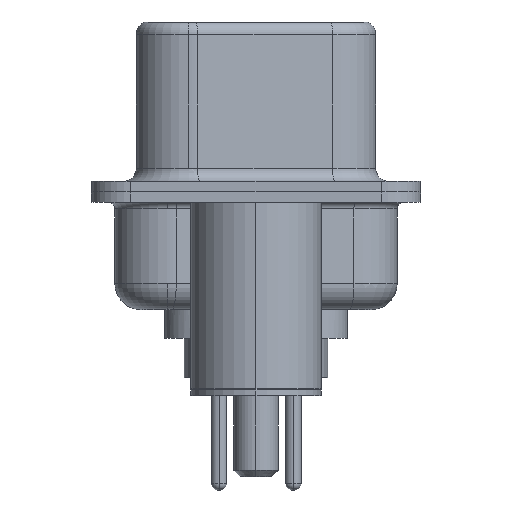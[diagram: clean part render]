
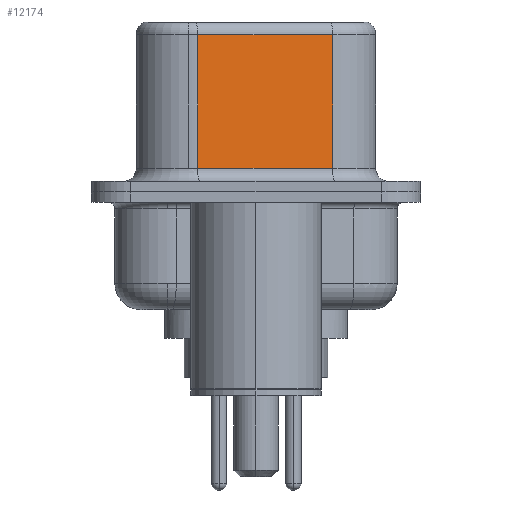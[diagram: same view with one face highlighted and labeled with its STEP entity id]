
A CAD part, left-side view. The second image highlights one B-rep face of the part: STEP entity #12174.
In plain terms, the highlighted planar face has unit normal (-0.985, -0.174, 0).
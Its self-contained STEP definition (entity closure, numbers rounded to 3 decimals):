
#230 = DIRECTION ( 'NONE',  ( 0.174, -0.985, 0. ) ) ;
#518 = CARTESIAN_POINT ( 'NONE',  ( 3.655, 2.233, 0.9 ) ) ;
#593 = VERTEX_POINT ( 'NONE', #15364 ) ;
#1044 = CARTESIAN_POINT ( 'NONE',  ( 4.565, -2.927, 6.02 ) ) ;
#1644 = CARTESIAN_POINT ( 'NONE',  ( 4.565, -2.927, 6.02 ) ) ;
#1929 = CARTESIAN_POINT ( 'NONE',  ( 3.655, 2.233, 6.02 ) ) ;
#2611 = ORIENTED_EDGE ( 'NONE', *, *, #14477, .T. ) ;
#2625 = CARTESIAN_POINT ( 'NONE',  ( 4.565, -2.927, 6.52 ) ) ;
#2682 = EDGE_CURVE ( 'NONE', #6691, #593, #7657, .T. ) ;
#3186 = ORIENTED_EDGE ( 'NONE', *, *, #2682, .F. ) ;
#3471 = AXIS2_PLACEMENT_3D ( 'NONE', #12317, #14825, #7135 ) ;
#3733 = DIRECTION ( 'NONE',  ( 0., 0., -1. ) ) ;
#3735 = LINE ( 'NONE', #7600, #13826 ) ;
#5850 = PLANE ( 'NONE',  #3471 ) ;
#6224 = VERTEX_POINT ( 'NONE', #1929 ) ;
#6691 = VERTEX_POINT ( 'NONE', #1644 ) ;
#7001 = DIRECTION ( 'NONE',  ( 0., 0., -1. ) ) ;
#7060 = EDGE_CURVE ( 'NONE', #6691, #6224, #7598, .T. ) ;
#7135 = DIRECTION ( 'NONE',  ( -0.174, 0.985, 0. ) ) ;
#7333 = VECTOR ( 'NONE', #7001, 1000. ) ;
#7438 = ORIENTED_EDGE ( 'NONE', *, *, #7060, .T. ) ;
#7598 = LINE ( 'NONE', #1044, #14048 ) ;
#7600 = CARTESIAN_POINT ( 'NONE',  ( 4.565, -2.927, 0.9 ) ) ;
#7657 = LINE ( 'NONE', #2625, #11150 ) ;
#9553 = VERTEX_POINT ( 'NONE', #518 ) ;
#10012 = EDGE_LOOP ( 'NONE', ( #3186, #7438, #10388, #2611 ) ) ;
#10388 = ORIENTED_EDGE ( 'NONE', *, *, #16082, .T. ) ;
#10830 = LINE ( 'NONE', #10886, #7333 ) ;
#10886 = CARTESIAN_POINT ( 'NONE',  ( 3.655, 2.233, 6.52 ) ) ;
#11150 = VECTOR ( 'NONE', #3733, 1000. ) ;
#11567 = FACE_OUTER_BOUND ( 'NONE', #10012, .T. ) ;
#12174 = ADVANCED_FACE ( 'NONE', ( #11567 ), #5850, .F. ) ;
#12317 = CARTESIAN_POINT ( 'NONE',  ( 4.565, -2.927, 6.52 ) ) ;
#13826 = VECTOR ( 'NONE', #230, 1000. ) ;
#14048 = VECTOR ( 'NONE', #16161, 1000. ) ;
#14477 = EDGE_CURVE ( 'NONE', #9553, #593, #3735, .T. ) ;
#14825 = DIRECTION ( 'NONE',  ( 0.985, 0.174, 0. ) ) ;
#15364 = CARTESIAN_POINT ( 'NONE',  ( 4.565, -2.927, 0.9 ) ) ;
#16082 = EDGE_CURVE ( 'NONE', #6224, #9553, #10830, .T. ) ;
#16161 = DIRECTION ( 'NONE',  ( -0.174, 0.985, 0. ) ) ;
